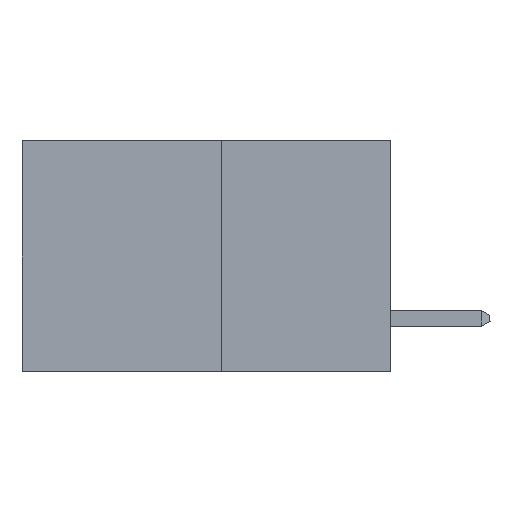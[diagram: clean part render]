
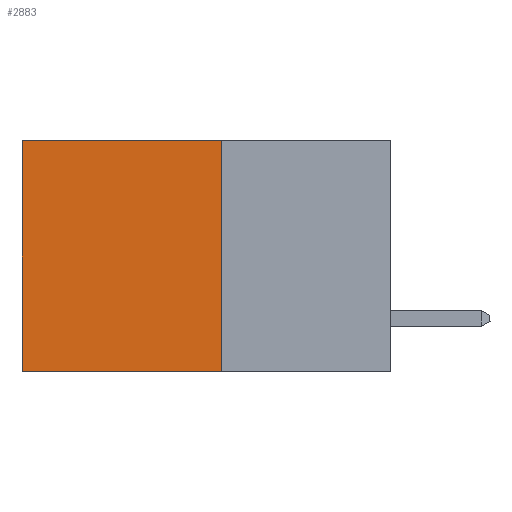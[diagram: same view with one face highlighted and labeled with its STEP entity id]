
A CAD part, left-side view. The second image highlights one B-rep face of the part: STEP entity #2883.
In plain terms, the highlighted planar face has unit normal (-1, 0, 0).
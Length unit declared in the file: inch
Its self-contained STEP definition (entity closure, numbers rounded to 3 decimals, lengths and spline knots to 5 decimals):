
#225 = VECTOR ( 'NONE', #15161, 39.37008 ) ;
#2452 = ORIENTED_EDGE ( 'NONE', *, *, #12457, .F. ) ;
#2702 = DIRECTION ( 'NONE',  ( 0., 0., -1. ) ) ;
#2751 = CARTESIAN_POINT ( 'NONE',  ( 0.277, 0.27, -0.37 ) ) ;
#2883 = ADVANCED_FACE ( 'NONE', ( #4248 ), #6150, .F. ) ;
#4214 = CARTESIAN_POINT ( 'NONE',  ( 0.277, 0.59, -0.37 ) ) ;
#4248 = FACE_OUTER_BOUND ( 'NONE', #9658, .T. ) ;
#4900 = CARTESIAN_POINT ( 'NONE',  ( 0.277, 0.27, 0. ) ) ;
#4973 = EDGE_CURVE ( 'NONE', #5020, #12072, #8647, .T. ) ;
#5020 = VERTEX_POINT ( 'NONE', #4900 ) ;
#5560 = VECTOR ( 'NONE', #8300, 39.37008 ) ;
#5800 = AXIS2_PLACEMENT_3D ( 'NONE', #14203, #6099, #2702 ) ;
#6099 = DIRECTION ( 'NONE',  ( 1., 0., 0. ) ) ;
#6150 = PLANE ( 'NONE',  #5800 ) ;
#6276 = EDGE_CURVE ( 'NONE', #12072, #10509, #9688, .T. ) ;
#6333 = DIRECTION ( 'NONE',  ( 0., 1., 0. ) ) ;
#6972 = VECTOR ( 'NONE', #6333, 39.37008 ) ;
#7120 = CARTESIAN_POINT ( 'NONE',  ( 0.277, 0.59, -0.37 ) ) ;
#7277 = CARTESIAN_POINT ( 'NONE',  ( 0.277, 0.59, 0. ) ) ;
#8300 = DIRECTION ( 'NONE',  ( 0., 1., 0. ) ) ;
#8647 = LINE ( 'NONE', #9420, #5560 ) ;
#9420 = CARTESIAN_POINT ( 'NONE',  ( 0.277, 0.27, 0. ) ) ;
#9422 = LINE ( 'NONE', #12566, #12492 ) ;
#9658 = EDGE_LOOP ( 'NONE', ( #11703, #12241, #2452, #10866 ) ) ;
#9688 = LINE ( 'NONE', #7120, #225 ) ;
#10069 = LINE ( 'NONE', #2751, #6972 ) ;
#10251 = DIRECTION ( 'NONE',  ( 0., 0., -1. ) ) ;
#10509 = VERTEX_POINT ( 'NONE', #4214 ) ;
#10866 = ORIENTED_EDGE ( 'NONE', *, *, #4973, .T. ) ;
#11703 = ORIENTED_EDGE ( 'NONE', *, *, #6276, .T. ) ;
#12072 = VERTEX_POINT ( 'NONE', #7277 ) ;
#12241 = ORIENTED_EDGE ( 'NONE', *, *, #14514, .F. ) ;
#12424 = CARTESIAN_POINT ( 'NONE',  ( 0.277, 0.27, -0.37 ) ) ;
#12457 = EDGE_CURVE ( 'NONE', #5020, #15191, #9422, .T. ) ;
#12492 = VECTOR ( 'NONE', #10251, 39.37008 ) ;
#12566 = CARTESIAN_POINT ( 'NONE',  ( 0.277, 0.27, -0.37 ) ) ;
#14203 = CARTESIAN_POINT ( 'NONE',  ( 0.277, 0.27, -0.37 ) ) ;
#14514 = EDGE_CURVE ( 'NONE', #15191, #10509, #10069, .T. ) ;
#15161 = DIRECTION ( 'NONE',  ( 0., 0., -1. ) ) ;
#15191 = VERTEX_POINT ( 'NONE', #12424 ) ;
